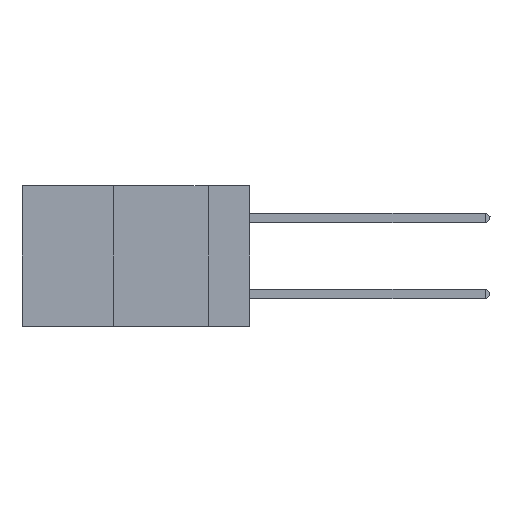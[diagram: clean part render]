
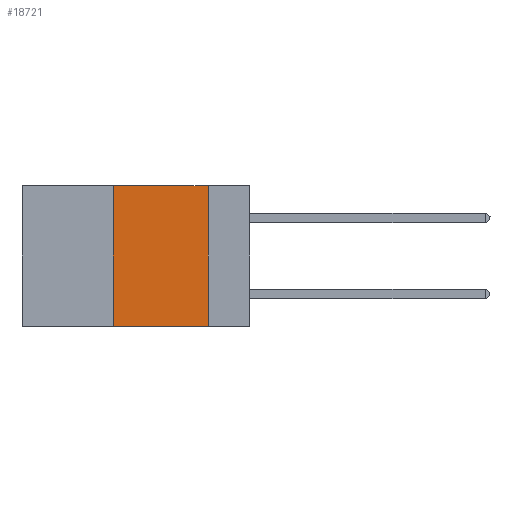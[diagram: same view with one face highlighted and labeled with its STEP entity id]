
A CAD part, left-side view. The second image highlights one B-rep face of the part: STEP entity #18721.
In plain terms, the highlighted planar face has unit normal (-1, 0, 0).
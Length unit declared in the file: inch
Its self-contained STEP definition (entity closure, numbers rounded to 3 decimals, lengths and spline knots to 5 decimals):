
#870 = CARTESIAN_POINT ( 'NONE',  ( 0., 0.11, 0. ) ) ;
#1206 = ORIENTED_EDGE ( 'NONE', *, *, #1741, .F. ) ;
#1411 = EDGE_CURVE ( 'NONE', #8103, #6968, #31060, .T. ) ;
#1741 = EDGE_CURVE ( 'NONE', #30940, #10816, #24976, .T. ) ;
#2938 = ORIENTED_EDGE ( 'NONE', *, *, #28357, .F. ) ;
#4159 = DIRECTION ( 'NONE',  ( 0., 0., -1. ) ) ;
#5464 = AXIS2_PLACEMENT_3D ( 'NONE', #26222, #39799, #40011 ) ;
#6968 = VERTEX_POINT ( 'NONE', #38117 ) ;
#7144 = LINE ( 'NONE', #15247, #27621 ) ;
#8103 = VERTEX_POINT ( 'NONE', #30576 ) ;
#10816 = VERTEX_POINT ( 'NONE', #21425 ) ;
#11965 = DIRECTION ( 'NONE',  ( 0., 0., 1. ) ) ;
#13145 = VECTOR ( 'NONE', #21867, 39.37008 ) ;
#15247 = CARTESIAN_POINT ( 'NONE',  ( 0., 0.36, 0. ) ) ;
#18721 = ADVANCED_FACE ( 'NONE', ( #22913 ), #35502, .F. ) ;
#18989 = CARTESIAN_POINT ( 'NONE',  ( 0., 0.6, 0. ) ) ;
#19998 = ORIENTED_EDGE ( 'NONE', *, *, #27303, .F. ) ;
#20834 = CARTESIAN_POINT ( 'NONE',  ( 0., 0.36, 0. ) ) ;
#21425 = CARTESIAN_POINT ( 'NONE',  ( 0., 0.11, 0. ) ) ;
#21568 = DIRECTION ( 'NONE',  ( 0., -1., 0. ) ) ;
#21867 = DIRECTION ( 'NONE',  ( 0., -1., 0. ) ) ;
#22913 = FACE_OUTER_BOUND ( 'NONE', #26765, .T. ) ;
#24976 = LINE ( 'NONE', #18989, #13145 ) ;
#25014 = VECTOR ( 'NONE', #21568, 39.37008 ) ;
#26222 = CARTESIAN_POINT ( 'NONE',  ( 0., 0.6, 0. ) ) ;
#26765 = EDGE_LOOP ( 'NONE', ( #2938, #1206, #19998, #37932 ) ) ;
#27303 = EDGE_CURVE ( 'NONE', #8103, #30940, #7144, .T. ) ;
#27621 = VECTOR ( 'NONE', #11965, 39.37008 ) ;
#27969 = CARTESIAN_POINT ( 'NONE',  ( 0., 0.6, -0.37 ) ) ;
#28357 = EDGE_CURVE ( 'NONE', #10816, #6968, #29111, .T. ) ;
#29111 = LINE ( 'NONE', #870, #34269 ) ;
#30576 = CARTESIAN_POINT ( 'NONE',  ( 0., 0.36, -0.37 ) ) ;
#30940 = VERTEX_POINT ( 'NONE', #20834 ) ;
#31060 = LINE ( 'NONE', #27969, #25014 ) ;
#34269 = VECTOR ( 'NONE', #4159, 39.37008 ) ;
#35502 = PLANE ( 'NONE',  #5464 ) ;
#37932 = ORIENTED_EDGE ( 'NONE', *, *, #1411, .T. ) ;
#38117 = CARTESIAN_POINT ( 'NONE',  ( 0., 0.11, -0.37 ) ) ;
#39799 = DIRECTION ( 'NONE',  ( 1., 0., 0. ) ) ;
#40011 = DIRECTION ( 'NONE',  ( 0., 0., -1. ) ) ;
